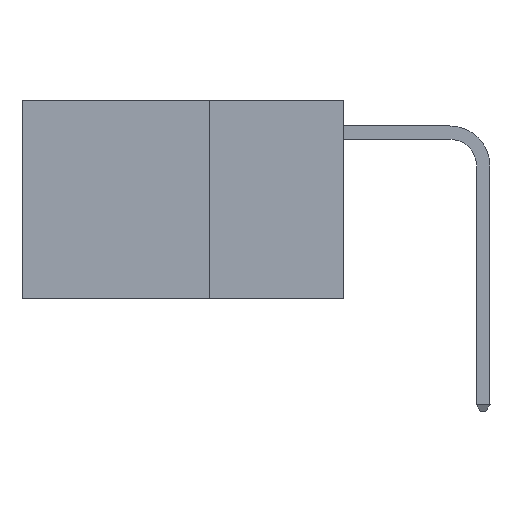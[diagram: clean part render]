
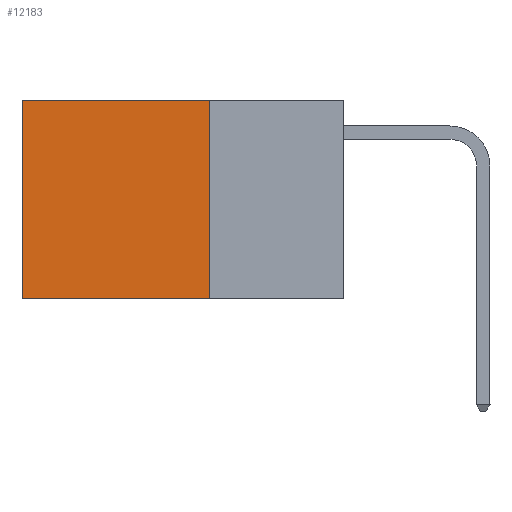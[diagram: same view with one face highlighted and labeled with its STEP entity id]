
A CAD part, left-side view. The second image highlights one B-rep face of the part: STEP entity #12183.
In plain terms, the highlighted planar face has unit normal (-1, 0, 0).
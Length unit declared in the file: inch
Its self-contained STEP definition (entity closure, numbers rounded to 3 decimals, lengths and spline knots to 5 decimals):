
#227 = CARTESIAN_POINT ( 'NONE',  ( 0.2625, 0.6, -0.37 ) ) ;
#688 = VERTEX_POINT ( 'NONE', #22172 ) ;
#1190 = CARTESIAN_POINT ( 'NONE',  ( 0.2625, 0.25, 0. ) ) ;
#1625 = EDGE_CURVE ( 'NONE', #688, #5715, #27734, .T. ) ;
#2338 = AXIS2_PLACEMENT_3D ( 'NONE', #4104, #3796, #13792 ) ;
#3796 = DIRECTION ( 'NONE',  ( 1., 0., 0. ) ) ;
#4104 = CARTESIAN_POINT ( 'NONE',  ( 0.2625, 0.25, 0. ) ) ;
#4876 = CARTESIAN_POINT ( 'NONE',  ( 0.2625, 0.25, 0. ) ) ;
#5581 = LINE ( 'NONE', #24852, #12138 ) ;
#5715 = VERTEX_POINT ( 'NONE', #30577 ) ;
#5876 = VERTEX_POINT ( 'NONE', #227 ) ;
#7396 = VECTOR ( 'NONE', #20719, 39.37008 ) ;
#7474 = VECTOR ( 'NONE', #21324, 39.37008 ) ;
#8882 = CARTESIAN_POINT ( 'NONE',  ( 0.2625, 0.25, -0.37 ) ) ;
#10809 = EDGE_CURVE ( 'NONE', #5715, #5876, #22932, .T. ) ;
#11389 = CARTESIAN_POINT ( 'NONE',  ( 0.2625, 0.6, 0. ) ) ;
#11695 = LINE ( 'NONE', #4876, #7474 ) ;
#12138 = VECTOR ( 'NONE', #25176, 39.37008 ) ;
#12183 = ADVANCED_FACE ( 'NONE', ( #23098 ), #13642, .F. ) ;
#12332 = ORIENTED_EDGE ( 'NONE', *, *, #1625, .T. ) ;
#13642 = PLANE ( 'NONE',  #2338 ) ;
#13792 = DIRECTION ( 'NONE',  ( 0., 0., -1. ) ) ;
#14692 = EDGE_CURVE ( 'NONE', #688, #17804, #11695, .T. ) ;
#15785 = EDGE_CURVE ( 'NONE', #17804, #5876, #5581, .T. ) ;
#15850 = ORIENTED_EDGE ( 'NONE', *, *, #14692, .F. ) ;
#17804 = VERTEX_POINT ( 'NONE', #8882 ) ;
#20338 = EDGE_LOOP ( 'NONE', ( #24776, #27174, #15850, #12332 ) ) ;
#20719 = DIRECTION ( 'NONE',  ( 0., 0., -1. ) ) ;
#21012 = VECTOR ( 'NONE', #27578, 39.37008 ) ;
#21324 = DIRECTION ( 'NONE',  ( 0., 0., -1. ) ) ;
#22172 = CARTESIAN_POINT ( 'NONE',  ( 0.2625, 0.25, 0. ) ) ;
#22932 = LINE ( 'NONE', #11389, #7396 ) ;
#23098 = FACE_OUTER_BOUND ( 'NONE', #20338, .T. ) ;
#24776 = ORIENTED_EDGE ( 'NONE', *, *, #10809, .T. ) ;
#24852 = CARTESIAN_POINT ( 'NONE',  ( 0.2625, 0.25, -0.37 ) ) ;
#25176 = DIRECTION ( 'NONE',  ( 0., 1., 0. ) ) ;
#27174 = ORIENTED_EDGE ( 'NONE', *, *, #15785, .F. ) ;
#27578 = DIRECTION ( 'NONE',  ( 0., 1., 0. ) ) ;
#27734 = LINE ( 'NONE', #1190, #21012 ) ;
#30577 = CARTESIAN_POINT ( 'NONE',  ( 0.2625, 0.6, 0. ) ) ;
